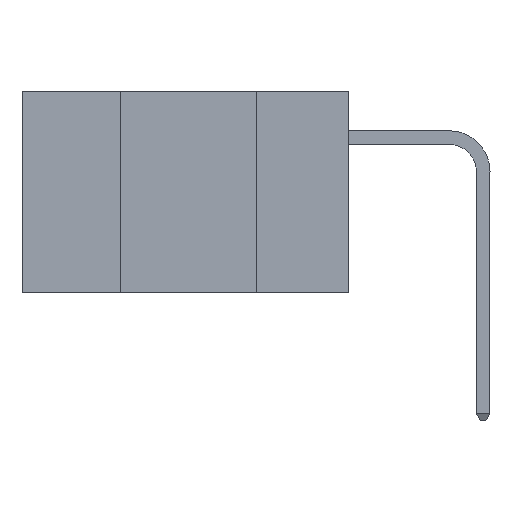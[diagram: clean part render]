
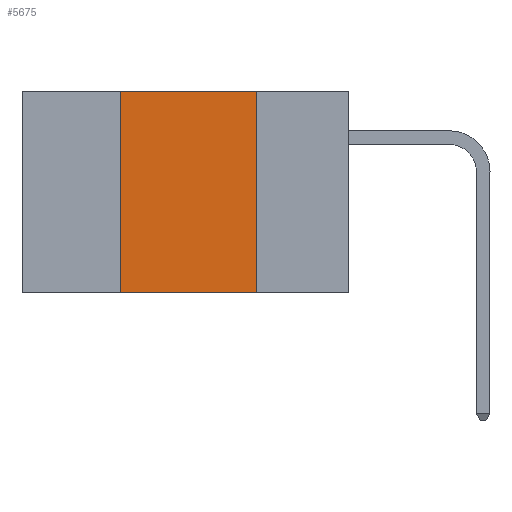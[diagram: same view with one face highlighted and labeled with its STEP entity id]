
A CAD part, left-side view. The second image highlights one B-rep face of the part: STEP entity #5675.
In plain terms, the highlighted planar face has unit normal (-1, 0, 0).
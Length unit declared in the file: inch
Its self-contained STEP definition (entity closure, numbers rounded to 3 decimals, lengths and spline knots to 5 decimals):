
#71 = LINE ( 'NONE', #3122, #12613 ) ;
#73 = CARTESIAN_POINT ( 'NONE',  ( 0., 0.6, 0. ) ) ;
#276 = ORIENTED_EDGE ( 'NONE', *, *, #8266, .T. ) ;
#495 = ORIENTED_EDGE ( 'NONE', *, *, #8034, .F. ) ;
#634 = CARTESIAN_POINT ( 'NONE',  ( 0., 0.17, 0. ) ) ;
#1815 = DIRECTION ( 'NONE',  ( 1., 0., 0. ) ) ;
#1843 = ORIENTED_EDGE ( 'NONE', *, *, #3840, .F. ) ;
#2121 = CARTESIAN_POINT ( 'NONE',  ( 0., 0.17, -0.37 ) ) ;
#2669 = CARTESIAN_POINT ( 'NONE',  ( 0., 0.42, 0. ) ) ;
#3122 = CARTESIAN_POINT ( 'NONE',  ( 0., 0.17, 0. ) ) ;
#3515 = LINE ( 'NONE', #2669, #3972 ) ;
#3656 = DIRECTION ( 'NONE',  ( 0., 0., 1. ) ) ;
#3840 = EDGE_CURVE ( 'NONE', #12260, #6890, #3515, .T. ) ;
#3972 = VECTOR ( 'NONE', #3656, 39.37008 ) ;
#4778 = VERTEX_POINT ( 'NONE', #2121 ) ;
#5675 = ADVANCED_FACE ( 'NONE', ( #6080 ), #9699, .F. ) ;
#5724 = LINE ( 'NONE', #6399, #7410 ) ;
#5755 = DIRECTION ( 'NONE',  ( 0., 0., -1. ) ) ;
#6080 = FACE_OUTER_BOUND ( 'NONE', #12011, .T. ) ;
#6399 = CARTESIAN_POINT ( 'NONE',  ( 0., 0.6, -0.37 ) ) ;
#6890 = VERTEX_POINT ( 'NONE', #7939 ) ;
#7198 = CARTESIAN_POINT ( 'NONE',  ( 0., 0.6, 0. ) ) ;
#7410 = VECTOR ( 'NONE', #8358, 39.37008 ) ;
#7560 = EDGE_CURVE ( 'NONE', #6890, #10545, #12347, .T. ) ;
#7939 = CARTESIAN_POINT ( 'NONE',  ( 0., 0.42, 0. ) ) ;
#8034 = EDGE_CURVE ( 'NONE', #10545, #4778, #71, .T. ) ;
#8176 = DIRECTION ( 'NONE',  ( 0., -1., 0. ) ) ;
#8266 = EDGE_CURVE ( 'NONE', #12260, #4778, #5724, .T. ) ;
#8358 = DIRECTION ( 'NONE',  ( 0., -1., 0. ) ) ;
#8975 = AXIS2_PLACEMENT_3D ( 'NONE', #73, #1815, #5755 ) ;
#9699 = PLANE ( 'NONE',  #8975 ) ;
#10389 = ORIENTED_EDGE ( 'NONE', *, *, #7560, .F. ) ;
#10545 = VERTEX_POINT ( 'NONE', #634 ) ;
#10805 = CARTESIAN_POINT ( 'NONE',  ( 0., 0.42, -0.37 ) ) ;
#10936 = DIRECTION ( 'NONE',  ( 0., 0., -1. ) ) ;
#11893 = VECTOR ( 'NONE', #8176, 39.37008 ) ;
#12011 = EDGE_LOOP ( 'NONE', ( #495, #10389, #1843, #276 ) ) ;
#12260 = VERTEX_POINT ( 'NONE', #10805 ) ;
#12347 = LINE ( 'NONE', #7198, #11893 ) ;
#12613 = VECTOR ( 'NONE', #10936, 39.37008 ) ;
